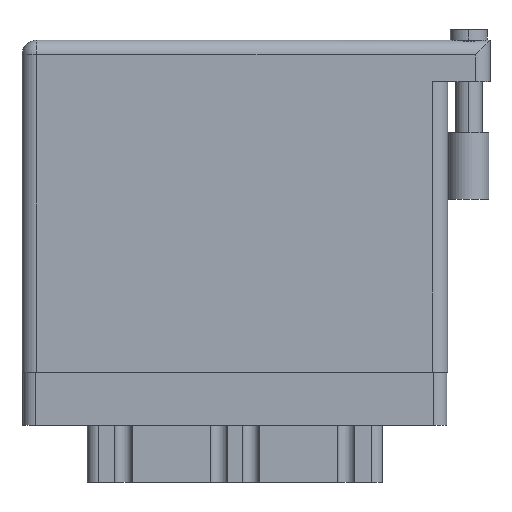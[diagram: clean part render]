
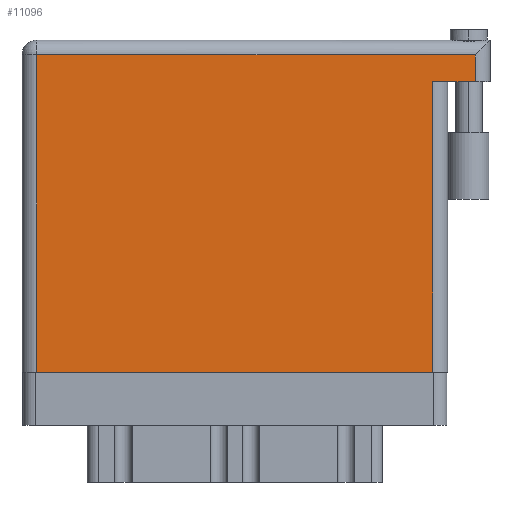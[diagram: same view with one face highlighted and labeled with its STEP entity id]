
A CAD part, front view. The second image highlights one B-rep face of the part: STEP entity #11096.
In plain terms, the highlighted face is planar.
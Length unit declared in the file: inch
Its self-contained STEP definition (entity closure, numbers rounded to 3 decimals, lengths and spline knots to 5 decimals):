
#16 = LINE ( 'NONE', #18447, #9167 ) ;
#162 = EDGE_CURVE ( 'NONE', #2214, #28194, #6484, .T. ) ;
#530 = CARTESIAN_POINT ( 'NONE',  ( 2.138, 1.369, 0. ) ) ;
#929 = AXIS2_PLACEMENT_3D ( 'NONE', #25113, #1304, #33113 ) ;
#1304 = DIRECTION ( 'NONE',  ( 0., 0., -1. ) ) ;
#2214 = VERTEX_POINT ( 'NONE', #30228 ) ;
#2859 = CARTESIAN_POINT ( 'NONE',  ( 1.938, 1.369, 0. ) ) ;
#2910 = CARTESIAN_POINT ( 'NONE',  ( 2.208, 1.369, 0. ) ) ;
#3207 = EDGE_CURVE ( 'NONE', #26581, #2214, #16, .T. ) ;
#3908 = EDGE_CURVE ( 'NONE', #4762, #25416, #26735, .T. ) ;
#4468 = DIRECTION ( 'NONE',  ( 0., 1., 0. ) ) ;
#4762 = VERTEX_POINT ( 'NONE', #530 ) ;
#4865 = EDGE_CURVE ( 'NONE', #4762, #26581, #6786, .T. ) ;
#6484 = LINE ( 'NONE', #21776, #27149 ) ;
#6786 = LINE ( 'NONE', #20346, #7488 ) ;
#7488 = VECTOR ( 'NONE', #12544, 39.37008 ) ;
#8033 = DIRECTION ( 'NONE',  ( -1., 0., 0. ) ) ;
#9067 = VERTEX_POINT ( 'NONE', #30023 ) ;
#9167 = VECTOR ( 'NONE', #8033, 39.37008 ) ;
#11096 = ADVANCED_FACE ( 'NONE', ( #22514 ), #27722, .F. ) ;
#12544 = DIRECTION ( 'NONE',  ( 0., 1., 0. ) ) ;
#12849 = ORIENTED_EDGE ( 'NONE', *, *, #14481, .T. ) ;
#13535 = DIRECTION ( 'NONE',  ( -1., 0., 0. ) ) ;
#13998 = ORIENTED_EDGE ( 'NONE', *, *, #162, .T. ) ;
#14230 = EDGE_LOOP ( 'NONE', ( #12849, #19650, #25424, #26256, #27842, #13998 ) ) ;
#14477 = DIRECTION ( 'NONE',  ( 0., -1., 0. ) ) ;
#14481 = EDGE_CURVE ( 'NONE', #28194, #9067, #34004, .T. ) ;
#14923 = LINE ( 'NONE', #25676, #21220 ) ;
#15669 = VECTOR ( 'NONE', #20965, 39.37008 ) ;
#16144 = CARTESIAN_POINT ( 'NONE',  ( 0.07, 0., 0. ) ) ;
#18447 = CARTESIAN_POINT ( 'NONE',  ( 0., 1.496, 0. ) ) ;
#19351 = EDGE_CURVE ( 'NONE', #9067, #25416, #14923, .T. ) ;
#19650 = ORIENTED_EDGE ( 'NONE', *, *, #19351, .T. ) ;
#20346 = CARTESIAN_POINT ( 'NONE',  ( 2.138, 1.566, 0. ) ) ;
#20965 = DIRECTION ( 'NONE',  ( 1., 0., 0. ) ) ;
#21220 = VECTOR ( 'NONE', #4468, 39.37008 ) ;
#21776 = CARTESIAN_POINT ( 'NONE',  ( 0.07, 0., 0. ) ) ;
#22514 = FACE_OUTER_BOUND ( 'NONE', #14230, .T. ) ;
#25113 = CARTESIAN_POINT ( 'NONE',  ( 0., 1.566, 0. ) ) ;
#25416 = VERTEX_POINT ( 'NONE', #2859 ) ;
#25424 = ORIENTED_EDGE ( 'NONE', *, *, #3908, .F. ) ;
#25676 = CARTESIAN_POINT ( 'NONE',  ( 1.938, 1.369, 0. ) ) ;
#26256 = ORIENTED_EDGE ( 'NONE', *, *, #4865, .T. ) ;
#26581 = VERTEX_POINT ( 'NONE', #34008 ) ;
#26735 = LINE ( 'NONE', #2910, #34089 ) ;
#27149 = VECTOR ( 'NONE', #14477, 39.37008 ) ;
#27722 = PLANE ( 'NONE',  #929 ) ;
#27842 = ORIENTED_EDGE ( 'NONE', *, *, #3207, .T. ) ;
#28194 = VERTEX_POINT ( 'NONE', #16144 ) ;
#30023 = CARTESIAN_POINT ( 'NONE',  ( 1.938, 0., 0. ) ) ;
#30228 = CARTESIAN_POINT ( 'NONE',  ( 0.07, 1.496, 0. ) ) ;
#31569 = CARTESIAN_POINT ( 'NONE',  ( 0., 0., 0. ) ) ;
#33113 = DIRECTION ( 'NONE',  ( -1., 0., 0. ) ) ;
#34004 = LINE ( 'NONE', #31569, #15669 ) ;
#34008 = CARTESIAN_POINT ( 'NONE',  ( 2.138, 1.496, 0. ) ) ;
#34089 = VECTOR ( 'NONE', #13535, 39.37008 ) ;
